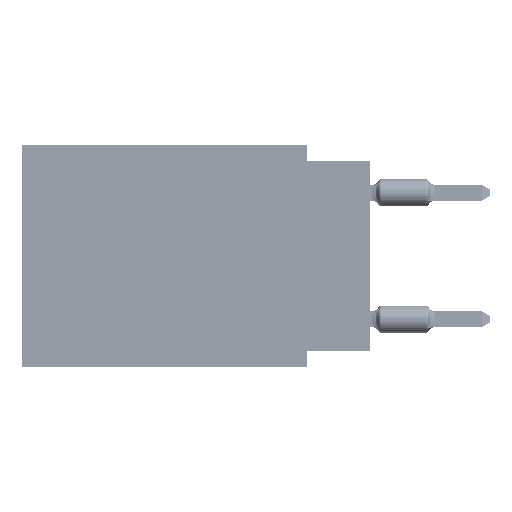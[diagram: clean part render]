
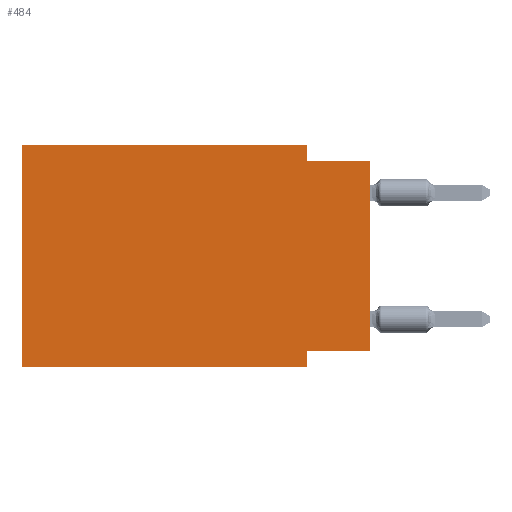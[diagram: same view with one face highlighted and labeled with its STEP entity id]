
A CAD part, left-side view. The second image highlights one B-rep face of the part: STEP entity #484.
In plain terms, the highlighted planar face has unit normal (-1, 0, 0).
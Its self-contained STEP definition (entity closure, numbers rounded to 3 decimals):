
#484 = ADVANCED_FACE ( 'NONE', ( #22783 ), #21613, .F. ) ;
#6462 = CARTESIAN_POINT ( 'NONE',  ( 0., 13.97, 0. ) ) ;
#6964 = EDGE_CURVE ( 'NONE', #73664, #62894, #26390, .T. ) ;
#7833 = ORIENTED_EDGE ( 'NONE', *, *, #6964, .F. ) ;
#11310 = CARTESIAN_POINT ( 'NONE',  ( 0., 2.54, 0. ) ) ;
#11405 = VERTEX_POINT ( 'NONE', #25260 ) ;
#11935 = VERTEX_POINT ( 'NONE', #32157 ) ;
#13098 = EDGE_CURVE ( 'NONE', #64739, #62894, #48833, .T. ) ;
#13611 = ORIENTED_EDGE ( 'NONE', *, *, #13098, .T. ) ;
#13667 = AXIS2_PLACEMENT_3D ( 'NONE', #69083, #46543, #33689 ) ;
#14639 = EDGE_CURVE ( 'NONE', #64739, #11935, #52783, .T. ) ;
#15786 = CARTESIAN_POINT ( 'NONE',  ( 0., 0., 0. ) ) ;
#17360 = DIRECTION ( 'NONE',  ( 0., 0., 1. ) ) ;
#18518 = DIRECTION ( 'NONE',  ( 0., 1., 0. ) ) ;
#19235 = ORIENTED_EDGE ( 'NONE', *, *, #38797, .T. ) ;
#20214 = EDGE_CURVE ( 'NONE', #41634, #46826, #63816, .T. ) ;
#21451 = ORIENTED_EDGE ( 'NONE', *, *, #35259, .F. ) ;
#21613 = PLANE ( 'NONE',  #13667 ) ;
#22783 = FACE_OUTER_BOUND ( 'NONE', #48290, .T. ) ;
#25260 = CARTESIAN_POINT ( 'NONE',  ( 0., 0., -0.635 ) ) ;
#26390 = LINE ( 'NONE', #67261, #50340 ) ;
#31280 = CARTESIAN_POINT ( 'NONE',  ( 0., 2.54, -8.255 ) ) ;
#31385 = ORIENTED_EDGE ( 'NONE', *, *, #56943, .F. ) ;
#32094 = ORIENTED_EDGE ( 'NONE', *, *, #20214, .F. ) ;
#32157 = CARTESIAN_POINT ( 'NONE',  ( 0., 13.97, 0. ) ) ;
#33310 = LINE ( 'NONE', #15786, #50140 ) ;
#33689 = DIRECTION ( 'NONE',  ( 0., 0., -1. ) ) ;
#35239 = CARTESIAN_POINT ( 'NONE',  ( 0., 0., -8.255 ) ) ;
#35259 = EDGE_CURVE ( 'NONE', #46826, #11405, #39876, .T. ) ;
#36050 = VECTOR ( 'NONE', #18518, 1000. ) ;
#38797 = EDGE_CURVE ( 'NONE', #65270, #11405, #33310, .T. ) ;
#39876 = LINE ( 'NONE', #44562, #63577 ) ;
#39890 = VECTOR ( 'NONE', #76574, 1000. ) ;
#40057 = VECTOR ( 'NONE', #17360, 1000. ) ;
#41634 = VERTEX_POINT ( 'NONE', #72905 ) ;
#44562 = CARTESIAN_POINT ( 'NONE',  ( 0., 0., -0.635 ) ) ;
#45168 = CARTESIAN_POINT ( 'NONE',  ( 0., 13.97, -8.89 ) ) ;
#46543 = DIRECTION ( 'NONE',  ( 1., 0., 0. ) ) ;
#46826 = VERTEX_POINT ( 'NONE', #58980 ) ;
#48290 = EDGE_LOOP ( 'NONE', ( #19235, #21451, #32094, #69413, #50793, #13611, #7833, #31385 ) ) ;
#48546 = CARTESIAN_POINT ( 'NONE',  ( 0., 13.97, 0. ) ) ;
#48833 = LINE ( 'NONE', #52871, #39890 ) ;
#50140 = VECTOR ( 'NONE', #62480, 1000. ) ;
#50340 = VECTOR ( 'NONE', #61431, 1000. ) ;
#50793 = ORIENTED_EDGE ( 'NONE', *, *, #14639, .F. ) ;
#52213 = CARTESIAN_POINT ( 'NONE',  ( 0., 2.54, -8.89 ) ) ;
#52783 = LINE ( 'NONE', #6462, #40057 ) ;
#52871 = CARTESIAN_POINT ( 'NONE',  ( 0., 13.97, -8.89 ) ) ;
#56943 = EDGE_CURVE ( 'NONE', #65270, #73664, #66739, .T. ) ;
#57597 = DIRECTION ( 'NONE',  ( 0., 0., -1. ) ) ;
#58023 = VECTOR ( 'NONE', #57597, 1000. ) ;
#58972 = VECTOR ( 'NONE', #72247, 1000. ) ;
#58980 = CARTESIAN_POINT ( 'NONE',  ( 0., 2.54, -0.635 ) ) ;
#61431 = DIRECTION ( 'NONE',  ( 0., 0., -1. ) ) ;
#62480 = DIRECTION ( 'NONE',  ( 0., 0., 1. ) ) ;
#62894 = VERTEX_POINT ( 'NONE', #52213 ) ;
#63212 = DIRECTION ( 'NONE',  ( 0., -1., 0. ) ) ;
#63577 = VECTOR ( 'NONE', #63212, 1000. ) ;
#63816 = LINE ( 'NONE', #11310, #58023 ) ;
#64739 = VERTEX_POINT ( 'NONE', #45168 ) ;
#65270 = VERTEX_POINT ( 'NONE', #35239 ) ;
#66739 = LINE ( 'NONE', #67118, #36050 ) ;
#67118 = CARTESIAN_POINT ( 'NONE',  ( 0., 0., -8.255 ) ) ;
#67261 = CARTESIAN_POINT ( 'NONE',  ( 0., 2.54, -8.89 ) ) ;
#69083 = CARTESIAN_POINT ( 'NONE',  ( 0., 13.97, 0. ) ) ;
#69413 = ORIENTED_EDGE ( 'NONE', *, *, #76251, .F. ) ;
#72247 = DIRECTION ( 'NONE',  ( 0., -1., 0. ) ) ;
#72905 = CARTESIAN_POINT ( 'NONE',  ( 0., 2.54, 0. ) ) ;
#73008 = LINE ( 'NONE', #48546, #58972 ) ;
#73664 = VERTEX_POINT ( 'NONE', #31280 ) ;
#76251 = EDGE_CURVE ( 'NONE', #11935, #41634, #73008, .T. ) ;
#76574 = DIRECTION ( 'NONE',  ( 0., -1., 0. ) ) ;
